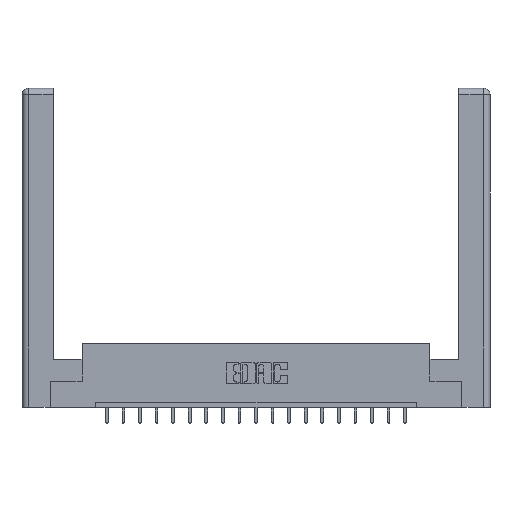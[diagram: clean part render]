
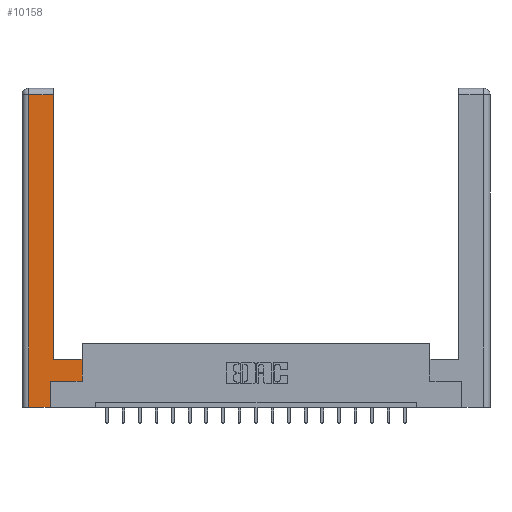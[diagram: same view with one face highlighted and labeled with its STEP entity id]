
A CAD part, top view. The second image highlights one B-rep face of the part: STEP entity #10158.
In plain terms, the highlighted planar face has unit normal (0, 0, 1).
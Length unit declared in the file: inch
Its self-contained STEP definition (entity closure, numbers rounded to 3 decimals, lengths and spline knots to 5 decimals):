
#48 = VECTOR ( 'NONE', #17322, 39.37008 ) ;
#336 = EDGE_CURVE ( 'NONE', #5377, #13110, #14466, .T. ) ;
#1154 = VERTEX_POINT ( 'NONE', #7329 ) ;
#1563 = CARTESIAN_POINT ( 'NONE',  ( 0.565, 0.245, 0. ) ) ;
#1602 = DIRECTION ( 'NONE',  ( 0., 1., 0. ) ) ;
#1765 = LINE ( 'NONE', #10379, #15614 ) ;
#1984 = EDGE_CURVE ( 'NONE', #13110, #1154, #11004, .T. ) ;
#2368 = VECTOR ( 'NONE', #11628, 39.37008 ) ;
#2416 = ORIENTED_EDGE ( 'NONE', *, *, #1984, .T. ) ;
#3295 = CARTESIAN_POINT ( 'NONE',  ( 0.565, 0.45, 0. ) ) ;
#3915 = ORIENTED_EDGE ( 'NONE', *, *, #15301, .T. ) ;
#4636 = VERTEX_POINT ( 'NONE', #7896 ) ;
#4796 = CARTESIAN_POINT ( 'NONE',  ( 0.295, 2.94, 0. ) ) ;
#4941 = DIRECTION ( 'NONE',  ( 0., 1., 0. ) ) ;
#5355 = EDGE_CURVE ( 'NONE', #4636, #18807, #1765, .T. ) ;
#5377 = VERTEX_POINT ( 'NONE', #17898 ) ;
#5501 = LINE ( 'NONE', #1563, #14639 ) ;
#6155 = CARTESIAN_POINT ( 'NONE',  ( 0.265, 0.245, 0. ) ) ;
#6367 = DIRECTION ( 'NONE',  ( 0., 1., 0. ) ) ;
#6636 = LINE ( 'NONE', #6155, #12869 ) ;
#7101 = DIRECTION ( 'NONE',  ( 0., -1., 0. ) ) ;
#7329 = CARTESIAN_POINT ( 'NONE',  ( 0.295, 0.45, 0. ) ) ;
#7860 = EDGE_LOOP ( 'NONE', ( #13251, #14106, #16054, #11215, #12513, #3915, #11300, #2416 ) ) ;
#7896 = CARTESIAN_POINT ( 'NONE',  ( 0.0615, 2.94, 0. ) ) ;
#8737 = VERTEX_POINT ( 'NONE', #4796 ) ;
#9165 = DIRECTION ( 'NONE',  ( 0., 0., -1. ) ) ;
#10158 = ADVANCED_FACE ( 'NONE', ( #17327 ), #11716, .F. ) ;
#10379 = CARTESIAN_POINT ( 'NONE',  ( 0.0615, 0., 0. ) ) ;
#10630 = DIRECTION ( 'NONE',  ( 1., 0., 0. ) ) ;
#10857 = VERTEX_POINT ( 'NONE', #17874 ) ;
#10900 = EDGE_CURVE ( 'NONE', #8737, #4636, #16674, .T. ) ;
#11004 = LINE ( 'NONE', #11208, #48 ) ;
#11208 = CARTESIAN_POINT ( 'NONE',  ( 0.295, 0.45, 0. ) ) ;
#11215 = ORIENTED_EDGE ( 'NONE', *, *, #11635, .T. ) ;
#11300 = ORIENTED_EDGE ( 'NONE', *, *, #336, .T. ) ;
#11422 = LINE ( 'NONE', #19762, #17857 ) ;
#11592 = EDGE_CURVE ( 'NONE', #10857, #12628, #6636, .T. ) ;
#11628 = DIRECTION ( 'NONE',  ( -1., 0., 0. ) ) ;
#11635 = EDGE_CURVE ( 'NONE', #18807, #10857, #11422, .T. ) ;
#11716 = PLANE ( 'NONE',  #12462 ) ;
#11752 = VECTOR ( 'NONE', #4941, 39.37008 ) ;
#12462 = AXIS2_PLACEMENT_3D ( 'NONE', #14787, #9165, #17961 ) ;
#12513 = ORIENTED_EDGE ( 'NONE', *, *, #11592, .T. ) ;
#12628 = VERTEX_POINT ( 'NONE', #18833 ) ;
#12869 = VECTOR ( 'NONE', #1602, 39.37008 ) ;
#13110 = VERTEX_POINT ( 'NONE', #18869 ) ;
#13251 = ORIENTED_EDGE ( 'NONE', *, *, #14928, .T. ) ;
#14106 = ORIENTED_EDGE ( 'NONE', *, *, #10900, .T. ) ;
#14466 = LINE ( 'NONE', #3295, #18018 ) ;
#14639 = VECTOR ( 'NONE', #17029, 39.37008 ) ;
#14787 = CARTESIAN_POINT ( 'NONE',  ( 0., 0., 0. ) ) ;
#14928 = EDGE_CURVE ( 'NONE', #1154, #8737, #15539, .T. ) ;
#15301 = EDGE_CURVE ( 'NONE', #12628, #5377, #5501, .T. ) ;
#15325 = CARTESIAN_POINT ( 'NONE',  ( 0.0615, 0., 0. ) ) ;
#15539 = LINE ( 'NONE', #17072, #11752 ) ;
#15614 = VECTOR ( 'NONE', #7101, 39.37008 ) ;
#16054 = ORIENTED_EDGE ( 'NONE', *, *, #5355, .T. ) ;
#16674 = LINE ( 'NONE', #19478, #2368 ) ;
#17029 = DIRECTION ( 'NONE',  ( 1., 0., 0. ) ) ;
#17072 = CARTESIAN_POINT ( 'NONE',  ( 0.295, 3., 0. ) ) ;
#17322 = DIRECTION ( 'NONE',  ( -1., 0., 0. ) ) ;
#17327 = FACE_OUTER_BOUND ( 'NONE', #7860, .T. ) ;
#17857 = VECTOR ( 'NONE', #10630, 39.37008 ) ;
#17874 = CARTESIAN_POINT ( 'NONE',  ( 0.265, 0., 0. ) ) ;
#17898 = CARTESIAN_POINT ( 'NONE',  ( 0.565, 0.245, 0. ) ) ;
#17961 = DIRECTION ( 'NONE',  ( -1., 0., 0. ) ) ;
#18018 = VECTOR ( 'NONE', #6367, 39.37008 ) ;
#18807 = VERTEX_POINT ( 'NONE', #15325 ) ;
#18833 = CARTESIAN_POINT ( 'NONE',  ( 0.265, 0.245, 0. ) ) ;
#18869 = CARTESIAN_POINT ( 'NONE',  ( 0.565, 0.45, 0. ) ) ;
#19478 = CARTESIAN_POINT ( 'NONE',  ( 0.0615, 2.94, 0. ) ) ;
#19762 = CARTESIAN_POINT ( 'NONE',  ( 0.265, 0., 0. ) ) ;
